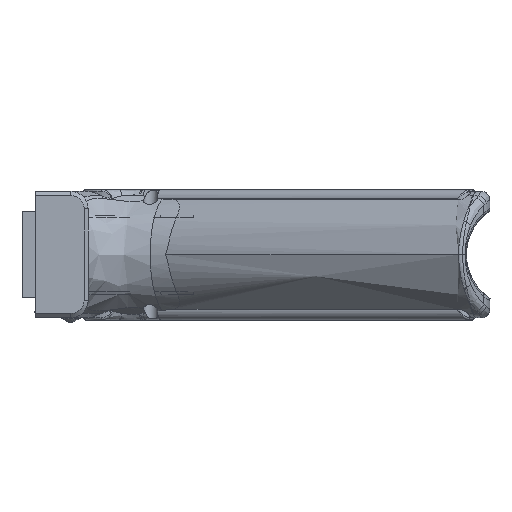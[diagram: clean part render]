
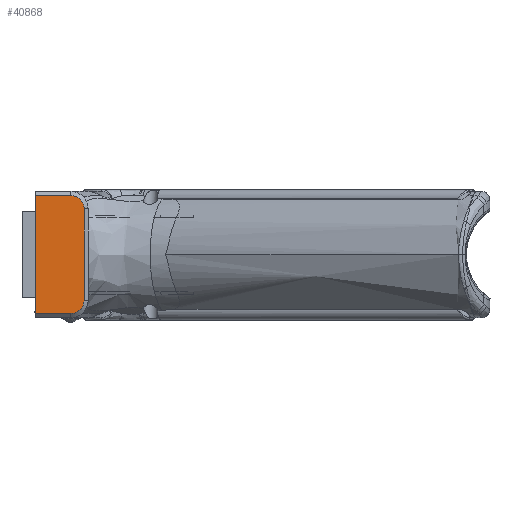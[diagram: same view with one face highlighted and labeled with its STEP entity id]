
A CAD part, left-side view. The second image highlights one B-rep face of the part: STEP entity #40868.
In plain terms, the highlighted planar face has unit normal (-1, 0, 0).
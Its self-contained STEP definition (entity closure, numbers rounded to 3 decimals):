
#1988=PLANE('',#42595);
#5175=FACE_OUTER_BOUND('',#7777,.T.);
#7777=EDGE_LOOP('',(#35697,#35698,#35699,#35700,#35701,#35702,#35703,#35704));
#9515=B_SPLINE_CURVE_WITH_KNOTS('',3,(#77613,#77614,#77615,#77616,#77617),
 .UNSPECIFIED.,.F.,.F.,(4,1,4),(-1.571,-0.898,0.),
 .UNSPECIFIED.);
#9517=B_SPLINE_CURVE_WITH_KNOTS('',3,(#77652,#77653,#77654,#77655,#77656),
 .UNSPECIFIED.,.F.,.F.,(4,1,4),(0.,0.673,
1.571),.UNSPECIFIED.);
#9519=B_SPLINE_CURVE_WITH_KNOTS('',3,(#77677,#77678,#77679,#77680),
 .UNSPECIFIED.,.F.,.F.,(4,4),(-0.41,-0.401),
 .UNSPECIFIED.);
#9521=B_SPLINE_CURVE_WITH_KNOTS('',3,(#77705,#77706,#77707,#77708),
 .UNSPECIFIED.,.F.,.F.,(4,4),(0.401,0.41),
 .UNSPECIFIED.);
#11733=LINE('',#69642,#14732);
#12181=LINE('',#77580,#15180);
#12185=LINE('',#77620,#15184);
#12190=LINE('',#77684,#15189);
#14732=VECTOR('',#46603,10.);
#15180=VECTOR('',#47747,10.);
#15184=VECTOR('',#47753,10.);
#15189=VECTOR('',#47760,10.);
#19274=VERTEX_POINT('',#69639);
#19275=VERTEX_POINT('',#69641);
#19534=VERTEX_POINT('',#77579);
#19535=VERTEX_POINT('',#77602);
#19538=VERTEX_POINT('',#77611);
#19539=VERTEX_POINT('',#77619);
#19541=VERTEX_POINT('',#77644);
#19543=VERTEX_POINT('',#77682);
#24313=EDGE_CURVE('',#19274,#19275,#11733,.T.);
#24997=EDGE_CURVE('',#19275,#19534,#12181,.T.);
#25002=EDGE_CURVE('',#19538,#19535,#9515,.T.);
#25003=EDGE_CURVE('',#19535,#19539,#12185,.T.);
#25008=EDGE_CURVE('',#19539,#19541,#9517,.T.);
#25010=EDGE_CURVE('',#19534,#19538,#9519,.T.);
#25012=EDGE_CURVE('',#19543,#19274,#12190,.T.);
#25014=EDGE_CURVE('',#19541,#19543,#9521,.T.);
#35697=ORIENTED_EDGE('',*,*,#24997,.F.);
#35698=ORIENTED_EDGE('',*,*,#24313,.F.);
#35699=ORIENTED_EDGE('',*,*,#25012,.F.);
#35700=ORIENTED_EDGE('',*,*,#25014,.F.);
#35701=ORIENTED_EDGE('',*,*,#25008,.F.);
#35702=ORIENTED_EDGE('',*,*,#25003,.F.);
#35703=ORIENTED_EDGE('',*,*,#25002,.F.);
#35704=ORIENTED_EDGE('',*,*,#25010,.F.);
#40868=ADVANCED_FACE('',(#5175),#1988,.T.);
#42595=AXIS2_PLACEMENT_3D('',#79598,#47976,#47977);
#46603=DIRECTION('',(0.,0.,1.));
#47747=DIRECTION('',(0.,-1.,0.));
#47753=DIRECTION('',(0.,0.,-1.));
#47760=DIRECTION('',(0.,1.,0.));
#47976=DIRECTION('center_axis',(-1.,0.,0.));
#47977=DIRECTION('ref_axis',(0.,-1.,0.));
#69639=CARTESIAN_POINT('',(-51.085,-1.479,-88.4));
#69641=CARTESIAN_POINT('',(-51.085,-1.479,-61.6));
#69642=CARTESIAN_POINT('',(-51.085,-1.479,-89.4));
#77579=CARTESIAN_POINT('',(-51.085,-9.53,-61.6));
#77580=CARTESIAN_POINT('',(-51.085,-4.516,-61.6));
#77602=CARTESIAN_POINT('',(-51.085,-12.629,-64.6));
#77611=CARTESIAN_POINT('',(-51.085,-9.614,-61.6));
#77613=CARTESIAN_POINT('Ctrl Pts',(-51.085,-9.614,-61.6));
#77614=CARTESIAN_POINT('Ctrl Pts',(-51.085,-10.292,-61.6));
#77615=CARTESIAN_POINT('Ctrl Pts',(-51.085,-11.874,
-62.15));
#77616=CARTESIAN_POINT('Ctrl Pts',(-51.085,-12.629,
-63.703));
#77617=CARTESIAN_POINT('Ctrl Pts',(-51.085,-12.629,-64.6));
#77619=CARTESIAN_POINT('',(-51.085,-12.629,-85.4));
#77620=CARTESIAN_POINT('',(-51.085,-12.629,-89.4));
#77644=CARTESIAN_POINT('',(-51.085,-9.614,-88.4));
#77652=CARTESIAN_POINT('Ctrl Pts',(-51.085,-12.629,
-85.4));
#77653=CARTESIAN_POINT('Ctrl Pts',(-51.085,-12.629,
-86.072));
#77654=CARTESIAN_POINT('Ctrl Pts',(-51.085,-12.079,
-87.644));
#77655=CARTESIAN_POINT('Ctrl Pts',(-51.085,-10.517,
-88.4));
#77656=CARTESIAN_POINT('Ctrl Pts',(-51.085,-9.614,
-88.4));
#77677=CARTESIAN_POINT('Ctrl Pts',(-51.085,-9.53,-61.6));
#77678=CARTESIAN_POINT('Ctrl Pts',(-51.085,-9.558,-61.6));
#77679=CARTESIAN_POINT('Ctrl Pts',(-51.085,-9.586,-61.6));
#77680=CARTESIAN_POINT('Ctrl Pts',(-51.085,-9.614,-61.6));
#77682=CARTESIAN_POINT('',(-51.085,-9.53,-88.4));
#77684=CARTESIAN_POINT('',(-51.085,-4.516,-88.4));
#77705=CARTESIAN_POINT('Ctrl Pts',(-51.085,-9.614,
-88.4));
#77706=CARTESIAN_POINT('Ctrl Pts',(-51.085,-9.586,-88.4));
#77707=CARTESIAN_POINT('Ctrl Pts',(-51.085,-9.558,
-88.4));
#77708=CARTESIAN_POINT('Ctrl Pts',(-51.085,-9.53,
-88.4));
#79598=CARTESIAN_POINT('Origin',(-51.085,-1.479,-89.4));
